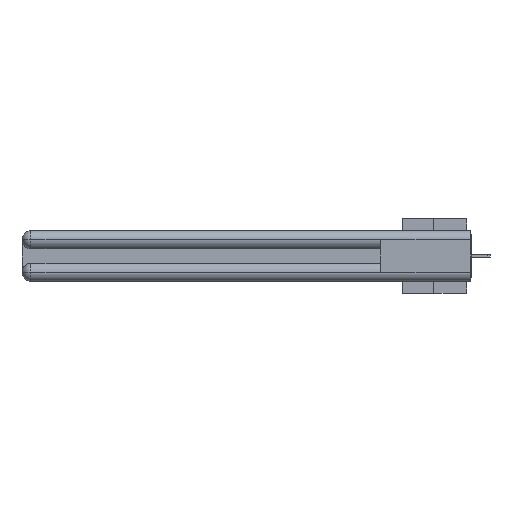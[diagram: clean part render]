
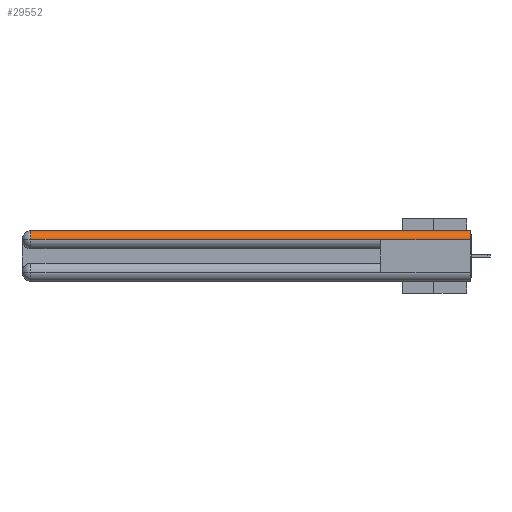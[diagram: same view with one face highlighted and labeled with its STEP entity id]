
A CAD part, left-side view. The second image highlights one B-rep face of the part: STEP entity #29552.
In plain terms, the highlighted cylindrical face has radius 1.562 mm (diameter 3.124 mm), a partial arc.
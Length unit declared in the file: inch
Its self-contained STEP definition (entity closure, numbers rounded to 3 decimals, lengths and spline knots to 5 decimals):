
#249 = DIRECTION ( 'NONE',  ( 0., 0., 1. ) ) ;
#279 = CARTESIAN_POINT ( 'NONE',  ( 0.0615, 0., 0. ) ) ;
#1553 = EDGE_CURVE ( 'NONE', #27786, #7880, #12742, .T. ) ;
#3188 = CARTESIAN_POINT ( 'NONE',  ( 0.0615, 0., -0.0615 ) ) ;
#3422 = DIRECTION ( 'NONE',  ( 0., -1., 0. ) ) ;
#3893 = CIRCLE ( 'NONE', #20273, 0.0615 ) ;
#4077 = VERTEX_POINT ( 'NONE', #13161 ) ;
#4874 = CYLINDRICAL_SURFACE ( 'NONE', #32503, 0.0615 ) ;
#6551 = ORIENTED_EDGE ( 'NONE', *, *, #1553, .F. ) ;
#7880 = VERTEX_POINT ( 'NONE', #32336 ) ;
#8757 = VECTOR ( 'NONE', #3422, 39.37008 ) ;
#9218 = EDGE_CURVE ( 'NONE', #27786, #4077, #30440, .T. ) ;
#9563 = CARTESIAN_POINT ( 'NONE',  ( 0., 0.6, -0.0615 ) ) ;
#9695 = CARTESIAN_POINT ( 'NONE',  ( 0., 0., -0.0615 ) ) ;
#10662 = VECTOR ( 'NONE', #18320, 39.37008 ) ;
#10838 = ORIENTED_EDGE ( 'NONE', *, *, #23173, .F. ) ;
#12377 = VERTEX_POINT ( 'NONE', #9695 ) ;
#12742 = LINE ( 'NONE', #279, #24035 ) ;
#13161 = CARTESIAN_POINT ( 'NONE',  ( 0., 2.94, -0.0615 ) ) ;
#13585 = DIRECTION ( 'NONE',  ( 1., 0., 0. ) ) ;
#13741 = DIRECTION ( 'NONE',  ( 0., -1., 0. ) ) ;
#17875 = EDGE_CURVE ( 'NONE', #12377, #25442, #21215, .T. ) ;
#18320 = DIRECTION ( 'NONE',  ( 0., 1., 0. ) ) ;
#18788 = CARTESIAN_POINT ( 'NONE',  ( 0., 3., -0.0615 ) ) ;
#18994 = AXIS2_PLACEMENT_3D ( 'NONE', #26530, #31809, #249 ) ;
#19866 = ORIENTED_EDGE ( 'NONE', *, *, #22303, .T. ) ;
#20222 = DIRECTION ( 'NONE',  ( 0., 0., 1. ) ) ;
#20273 = AXIS2_PLACEMENT_3D ( 'NONE', #3188, #28938, #13585 ) ;
#20572 = FACE_OUTER_BOUND ( 'NONE', #32995, .T. ) ;
#21215 = LINE ( 'NONE', #26651, #10662 ) ;
#22303 = EDGE_CURVE ( 'NONE', #4077, #25442, #31247, .T. ) ;
#23173 = EDGE_CURVE ( 'NONE', #7880, #12377, #3893, .T. ) ;
#24035 = VECTOR ( 'NONE', #13741, 39.37008 ) ;
#24668 = ORIENTED_EDGE ( 'NONE', *, *, #9218, .T. ) ;
#25442 = VERTEX_POINT ( 'NONE', #9563 ) ;
#26187 = DIRECTION ( 'NONE',  ( 0., 1., 0. ) ) ;
#26530 = CARTESIAN_POINT ( 'NONE',  ( 0.0615, 2.94, -0.0615 ) ) ;
#26651 = CARTESIAN_POINT ( 'NONE',  ( 0., 3., -0.0615 ) ) ;
#27786 = VERTEX_POINT ( 'NONE', #31285 ) ;
#28742 = CARTESIAN_POINT ( 'NONE',  ( 0.0615, 0., -0.0615 ) ) ;
#28938 = DIRECTION ( 'NONE',  ( 0., -1., 0. ) ) ;
#29330 = ORIENTED_EDGE ( 'NONE', *, *, #17875, .F. ) ;
#29552 = ADVANCED_FACE ( 'NONE', ( #20572 ), #4874, .T. ) ;
#30440 = CIRCLE ( 'NONE', #18994, 0.0615 ) ;
#31247 = LINE ( 'NONE', #18788, #8757 ) ;
#31285 = CARTESIAN_POINT ( 'NONE',  ( 0.0615, 2.94, 0. ) ) ;
#31809 = DIRECTION ( 'NONE',  ( 0., -1., 0. ) ) ;
#32336 = CARTESIAN_POINT ( 'NONE',  ( 0.0615, 0., 0. ) ) ;
#32503 = AXIS2_PLACEMENT_3D ( 'NONE', #28742, #26187, #20222 ) ;
#32995 = EDGE_LOOP ( 'NONE', ( #6551, #24668, #19866, #29330, #10838 ) ) ;
